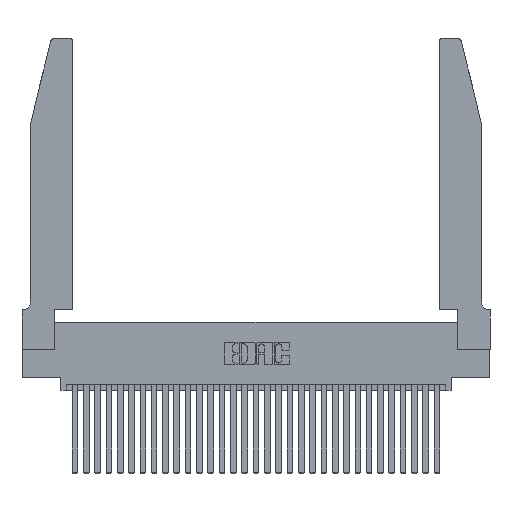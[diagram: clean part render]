
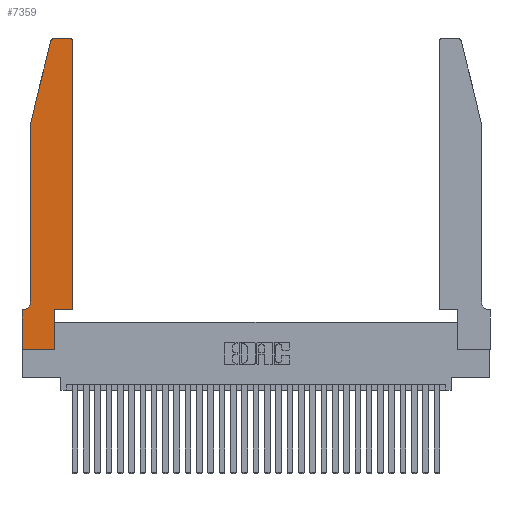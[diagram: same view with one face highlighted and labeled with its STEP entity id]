
A CAD part, top view. The second image highlights one B-rep face of the part: STEP entity #7359.
In plain terms, the highlighted planar face has unit normal (0, 0, 1).
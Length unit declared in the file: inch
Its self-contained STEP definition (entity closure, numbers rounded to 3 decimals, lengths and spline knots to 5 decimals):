
#58 = VECTOR ( 'NONE', #21935, 39.37008 ) ;
#238 = LINE ( 'NONE', #21068, #10704 ) ;
#387 = CARTESIAN_POINT ( 'NONE',  ( 0.0755, 2., 0.37 ) ) ;
#515 = VECTOR ( 'NONE', #16302, 39.37008 ) ;
#873 = CARTESIAN_POINT ( 'NONE',  ( 0.0755, 2., 0.37 ) ) ;
#911 = DIRECTION ( 'NONE',  ( 1., 0., 0. ) ) ;
#1956 = CARTESIAN_POINT ( 'NONE',  ( 0.0055, 0.42, 0.37 ) ) ;
#3205 = VERTEX_POINT ( 'NONE', #22832 ) ;
#3264 = VERTEX_POINT ( 'NONE', #12400 ) ;
#3404 = VERTEX_POINT ( 'NONE', #5900 ) ;
#4002 = ORIENTED_EDGE ( 'NONE', *, *, #6544, .T. ) ;
#4358 = ORIENTED_EDGE ( 'NONE', *, *, #18022, .T. ) ;
#4512 = ORIENTED_EDGE ( 'NONE', *, *, #27832, .T. ) ;
#4659 = CARTESIAN_POINT ( 'NONE',  ( 0., 0., 0.37 ) ) ;
#4749 = EDGE_CURVE ( 'NONE', #3404, #19203, #26308, .T. ) ;
#5291 = VERTEX_POINT ( 'NONE', #10891 ) ;
#5558 = VERTEX_POINT ( 'NONE', #24162 ) ;
#5900 = CARTESIAN_POINT ( 'NONE',  ( 0.4505, 0.35, 0.37 ) ) ;
#6000 = CARTESIAN_POINT ( 'NONE',  ( 0., 0.35, 0.37 ) ) ;
#6087 = CARTESIAN_POINT ( 'NONE',  ( 0.284, 2.75, 0.37 ) ) ;
#6311 = ORIENTED_EDGE ( 'NONE', *, *, #25528, .T. ) ;
#6389 = VERTEX_POINT ( 'NONE', #17588 ) ;
#6544 = EDGE_CURVE ( 'NONE', #5291, #25763, #28866, .T. ) ;
#7193 = ORIENTED_EDGE ( 'NONE', *, *, #25225, .T. ) ;
#7359 = ADVANCED_FACE ( 'NONE', ( #7727 ), #8702, .T. ) ;
#7727 = FACE_OUTER_BOUND ( 'NONE', #28975, .T. ) ;
#7996 = EDGE_CURVE ( 'NONE', #25763, #6389, #14625, .T. ) ;
#8075 = VECTOR ( 'NONE', #25509, 39.37008 ) ;
#8540 = CARTESIAN_POINT ( 'NONE',  ( 0.4505, 0.35, 0.37 ) ) ;
#8558 = CIRCLE ( 'NONE', #18354, 0.03 ) ;
#8619 = VECTOR ( 'NONE', #26777, 39.37008 ) ;
#8702 = PLANE ( 'NONE',  #16838 ) ;
#8779 = CARTESIAN_POINT ( 'NONE',  ( 0.4505, 2.72, 0.37 ) ) ;
#8965 = ORIENTED_EDGE ( 'NONE', *, *, #13859, .T. ) ;
#9370 = CARTESIAN_POINT ( 'NONE',  ( 0.4505, 0.35, 0.37 ) ) ;
#10031 = ORIENTED_EDGE ( 'NONE', *, *, #23602, .T. ) ;
#10343 = DIRECTION ( 'NONE',  ( 0., 0., 1. ) ) ;
#10704 = VECTOR ( 'NONE', #16674, 39.37008 ) ;
#10772 = CIRCLE ( 'NONE', #29267, 0.03 ) ;
#10891 = CARTESIAN_POINT ( 'NONE',  ( 0.25487, 2.72718, 0.37 ) ) ;
#11106 = CARTESIAN_POINT ( 'NONE',  ( 0.0755, 2., 0.37 ) ) ;
#11629 = VERTEX_POINT ( 'NONE', #12213 ) ;
#12121 = ORIENTED_EDGE ( 'NONE', *, *, #7996, .T. ) ;
#12164 = DIRECTION ( 'NONE',  ( 1., 0., 0. ) ) ;
#12213 = CARTESIAN_POINT ( 'NONE',  ( 0.0055, 0.35, 0.37 ) ) ;
#12400 = CARTESIAN_POINT ( 'NONE',  ( 0.2865, 0., 0.37 ) ) ;
#13213 = VECTOR ( 'NONE', #12164, 39.37008 ) ;
#13551 = DIRECTION ( 'NONE',  ( 1., 0., 0. ) ) ;
#13564 = DIRECTION ( 'NONE',  ( -0.239, -0.971, 0. ) ) ;
#13722 = CARTESIAN_POINT ( 'NONE',  ( 0.2865, 0.35, 0.37 ) ) ;
#13734 = LINE ( 'NONE', #29970, #30202 ) ;
#13859 = EDGE_CURVE ( 'NONE', #6389, #11629, #22060, .T. ) ;
#14625 = LINE ( 'NONE', #873, #8075 ) ;
#15920 = DIRECTION ( 'NONE',  ( 0., 0., 1. ) ) ;
#15940 = LINE ( 'NONE', #4659, #8619 ) ;
#16302 = DIRECTION ( 'NONE',  ( 0., 1., 0. ) ) ;
#16489 = ORIENTED_EDGE ( 'NONE', *, *, #29851, .T. ) ;
#16571 = AXIS2_PLACEMENT_3D ( 'NONE', #1956, #19023, #23707 ) ;
#16674 = DIRECTION ( 'NONE',  ( -1., 0., 0. ) ) ;
#16838 = AXIS2_PLACEMENT_3D ( 'NONE', #6000, #15920, #13551 ) ;
#17051 = ORIENTED_EDGE ( 'NONE', *, *, #4749, .T. ) ;
#17588 = CARTESIAN_POINT ( 'NONE',  ( 0.0755, 0.42, 0.37 ) ) ;
#17881 = VERTEX_POINT ( 'NONE', #6087 ) ;
#18022 = EDGE_CURVE ( 'NONE', #3264, #22545, #31648, .T. ) ;
#18354 = AXIS2_PLACEMENT_3D ( 'NONE', #20633, #10343, #22748 ) ;
#19023 = DIRECTION ( 'NONE',  ( 0., 0., -1. ) ) ;
#19203 = VERTEX_POINT ( 'NONE', #8779 ) ;
#19267 = EDGE_CURVE ( 'NONE', #11629, #3205, #22359, .T. ) ;
#20633 = CARTESIAN_POINT ( 'NONE',  ( 0.284, 2.72, 0.37 ) ) ;
#20833 = DIRECTION ( 'NONE',  ( 0., 0., 1. ) ) ;
#21068 = CARTESIAN_POINT ( 'NONE',  ( 0.2605, 2.75, 0.37 ) ) ;
#21219 = VECTOR ( 'NONE', #13564, 39.37008 ) ;
#21935 = DIRECTION ( 'NONE',  ( -1., 0., 0. ) ) ;
#22060 = CIRCLE ( 'NONE', #16571, 0.07 ) ;
#22359 = LINE ( 'NONE', #31276, #58 ) ;
#22545 = VERTEX_POINT ( 'NONE', #13722 ) ;
#22686 = DIRECTION ( 'NONE',  ( 0., -1., 0. ) ) ;
#22748 = DIRECTION ( 'NONE',  ( 1., 0., 0. ) ) ;
#22832 = CARTESIAN_POINT ( 'NONE',  ( 0., 0.35, 0.37 ) ) ;
#23386 = CARTESIAN_POINT ( 'NONE',  ( 0.2865, 0.35, 0.37 ) ) ;
#23402 = CARTESIAN_POINT ( 'NONE',  ( 0.4205, 2.72, 0.37 ) ) ;
#23602 = EDGE_CURVE ( 'NONE', #17881, #5291, #8558, .T. ) ;
#23707 = DIRECTION ( 'NONE',  ( -1., 0., 0. ) ) ;
#23916 = CARTESIAN_POINT ( 'NONE',  ( 0.4205, 2.75, 0.37 ) ) ;
#24162 = CARTESIAN_POINT ( 'NONE',  ( 0., 0., 0.37 ) ) ;
#24782 = VECTOR ( 'NONE', #25692, 39.37008 ) ;
#25225 = EDGE_CURVE ( 'NONE', #3205, #5558, #13734, .T. ) ;
#25509 = DIRECTION ( 'NONE',  ( 0., -1., 0. ) ) ;
#25528 = EDGE_CURVE ( 'NONE', #28229, #17881, #238, .T. ) ;
#25692 = DIRECTION ( 'NONE',  ( 0., 1., 0. ) ) ;
#25763 = VERTEX_POINT ( 'NONE', #387 ) ;
#26308 = LINE ( 'NONE', #8540, #24782 ) ;
#26777 = DIRECTION ( 'NONE',  ( 1., 0., 0. ) ) ;
#27362 = LINE ( 'NONE', #9370, #13213 ) ;
#27426 = EDGE_CURVE ( 'NONE', #5558, #3264, #15940, .T. ) ;
#27832 = EDGE_CURVE ( 'NONE', #22545, #3404, #27362, .T. ) ;
#27863 = ORIENTED_EDGE ( 'NONE', *, *, #27426, .T. ) ;
#28229 = VERTEX_POINT ( 'NONE', #23916 ) ;
#28726 = ORIENTED_EDGE ( 'NONE', *, *, #19267, .T. ) ;
#28866 = LINE ( 'NONE', #11106, #21219 ) ;
#28975 = EDGE_LOOP ( 'NONE', ( #6311, #10031, #4002, #12121, #8965, #28726, #7193, #27863, #4358, #4512, #17051, #16489 ) ) ;
#29267 = AXIS2_PLACEMENT_3D ( 'NONE', #23402, #20833, #911 ) ;
#29851 = EDGE_CURVE ( 'NONE', #19203, #28229, #10772, .T. ) ;
#29970 = CARTESIAN_POINT ( 'NONE',  ( 0., 0., 0.37 ) ) ;
#30202 = VECTOR ( 'NONE', #22686, 39.37008 ) ;
#31276 = CARTESIAN_POINT ( 'NONE',  ( 0.0755, 0.35, 0.37 ) ) ;
#31648 = LINE ( 'NONE', #23386, #515 ) ;
